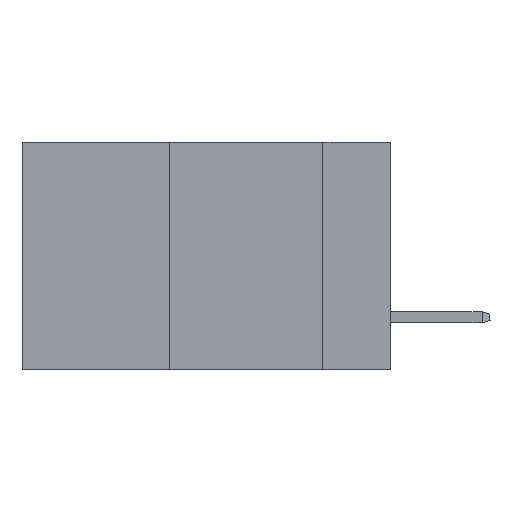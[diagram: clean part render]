
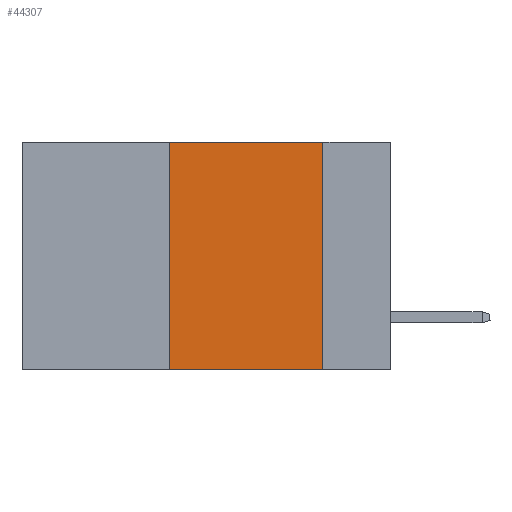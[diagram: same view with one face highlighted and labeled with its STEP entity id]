
A CAD part, left-side view. The second image highlights one B-rep face of the part: STEP entity #44307.
In plain terms, the highlighted planar face has unit normal (-1, 0, 0).
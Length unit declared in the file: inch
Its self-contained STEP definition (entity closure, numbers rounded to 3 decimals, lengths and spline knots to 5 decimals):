
#350 = CARTESIAN_POINT ( 'NONE',  ( 0., 0.11, -0.37 ) ) ;
#761 = DIRECTION ( 'NONE',  ( 1., 0., 0. ) ) ;
#887 = ORIENTED_EDGE ( 'NONE', *, *, #7813, .F. ) ;
#2324 = LINE ( 'NONE', #7136, #11512 ) ;
#4715 = PLANE ( 'NONE',  #39748 ) ;
#7136 = CARTESIAN_POINT ( 'NONE',  ( 0., 0.6, 0. ) ) ;
#7813 = EDGE_CURVE ( 'NONE', #21168, #12816, #28932, .T. ) ;
#10160 = DIRECTION ( 'NONE',  ( 0., -1., 0. ) ) ;
#10364 = CARTESIAN_POINT ( 'NONE',  ( 0., 0.11, 0. ) ) ;
#10872 = VECTOR ( 'NONE', #10160, 39.37008 ) ;
#11328 = FACE_OUTER_BOUND ( 'NONE', #22470, .T. ) ;
#11512 = VECTOR ( 'NONE', #46837, 39.37008 ) ;
#12816 = VERTEX_POINT ( 'NONE', #46767 ) ;
#21012 = CARTESIAN_POINT ( 'NONE',  ( 0., 0.6, 0. ) ) ;
#21168 = VERTEX_POINT ( 'NONE', #25491 ) ;
#22161 = VERTEX_POINT ( 'NONE', #350 ) ;
#22470 = EDGE_LOOP ( 'NONE', ( #36280, #34593, #887, #43999 ) ) ;
#23832 = LINE ( 'NONE', #42301, #10872 ) ;
#24258 = DIRECTION ( 'NONE',  ( 0., 0., 1. ) ) ;
#24450 = DIRECTION ( 'NONE',  ( 0., 0., -1. ) ) ;
#24618 = EDGE_CURVE ( 'NONE', #12816, #42832, #2324, .T. ) ;
#25491 = CARTESIAN_POINT ( 'NONE',  ( 0., 0.36, -0.37 ) ) ;
#28932 = LINE ( 'NONE', #47662, #49850 ) ;
#31742 = EDGE_CURVE ( 'NONE', #42832, #22161, #49350, .T. ) ;
#33659 = CARTESIAN_POINT ( 'NONE',  ( 0., 0.11, 0. ) ) ;
#34129 = EDGE_CURVE ( 'NONE', #21168, #22161, #23832, .T. ) ;
#34593 = ORIENTED_EDGE ( 'NONE', *, *, #24618, .F. ) ;
#36280 = ORIENTED_EDGE ( 'NONE', *, *, #31742, .F. ) ;
#37634 = DIRECTION ( 'NONE',  ( 0., 0., -1. ) ) ;
#38881 = VECTOR ( 'NONE', #37634, 39.37008 ) ;
#39748 = AXIS2_PLACEMENT_3D ( 'NONE', #21012, #761, #24450 ) ;
#42301 = CARTESIAN_POINT ( 'NONE',  ( 0., 0.6, -0.37 ) ) ;
#42832 = VERTEX_POINT ( 'NONE', #10364 ) ;
#43999 = ORIENTED_EDGE ( 'NONE', *, *, #34129, .T. ) ;
#44307 = ADVANCED_FACE ( 'NONE', ( #11328 ), #4715, .F. ) ;
#46767 = CARTESIAN_POINT ( 'NONE',  ( 0., 0.36, 0. ) ) ;
#46837 = DIRECTION ( 'NONE',  ( 0., -1., 0. ) ) ;
#47662 = CARTESIAN_POINT ( 'NONE',  ( 0., 0.36, 0. ) ) ;
#49350 = LINE ( 'NONE', #33659, #38881 ) ;
#49850 = VECTOR ( 'NONE', #24258, 39.37008 ) ;
